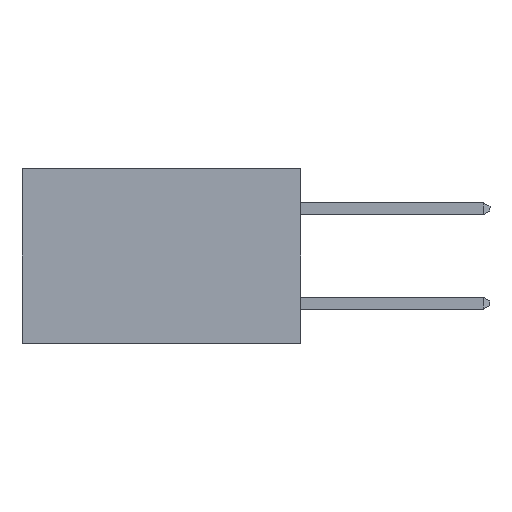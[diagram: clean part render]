
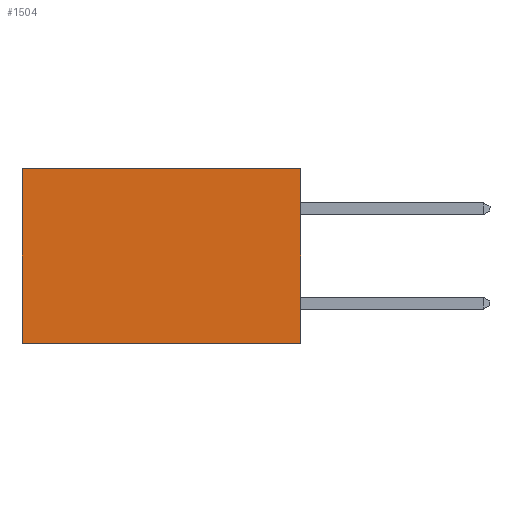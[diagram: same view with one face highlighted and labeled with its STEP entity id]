
A CAD part, left-side view. The second image highlights one B-rep face of the part: STEP entity #1504.
In plain terms, the highlighted planar face has unit normal (-1, 0, 0).
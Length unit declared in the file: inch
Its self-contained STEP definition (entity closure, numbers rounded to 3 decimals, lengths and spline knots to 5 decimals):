
#148 = VECTOR ( 'NONE', #6939, 39.37008 ) ;
#310 = VECTOR ( 'NONE', #2291, 39.37008 ) ;
#412 = ORIENTED_EDGE ( 'NONE', *, *, #3714, .T. ) ;
#515 = LINE ( 'NONE', #3896, #7092 ) ;
#741 = LINE ( 'NONE', #1169, #7304 ) ;
#976 = DIRECTION ( 'NONE',  ( 0., 1., 0. ) ) ;
#1053 = DIRECTION ( 'NONE',  ( 0., 0., -1. ) ) ;
#1169 = CARTESIAN_POINT ( 'NONE',  ( 0.277, 0., -0.37 ) ) ;
#1297 = DIRECTION ( 'NONE',  ( 0., 0., -1. ) ) ;
#1337 = DIRECTION ( 'NONE',  ( 1., 0., 0. ) ) ;
#1363 = PLANE ( 'NONE',  #7190 ) ;
#1504 = ADVANCED_FACE ( 'NONE', ( #4090 ), #1363, .F. ) ;
#1715 = CARTESIAN_POINT ( 'NONE',  ( 0.277, 0., -0.37 ) ) ;
#1769 = CARTESIAN_POINT ( 'NONE',  ( 0.277, 0., -0.37 ) ) ;
#1957 = EDGE_CURVE ( 'NONE', #2985, #2494, #741, .T. ) ;
#2291 = DIRECTION ( 'NONE',  ( 0., 1., 0. ) ) ;
#2494 = VERTEX_POINT ( 'NONE', #1769 ) ;
#2717 = VERTEX_POINT ( 'NONE', #8115 ) ;
#2786 = EDGE_CURVE ( 'NONE', #2717, #3017, #4804, .T. ) ;
#2985 = VERTEX_POINT ( 'NONE', #4842 ) ;
#3017 = VERTEX_POINT ( 'NONE', #4773 ) ;
#3580 = CARTESIAN_POINT ( 'NONE',  ( 0.277, 0., -0.37 ) ) ;
#3714 = EDGE_CURVE ( 'NONE', #2985, #2717, #515, .T. ) ;
#3896 = CARTESIAN_POINT ( 'NONE',  ( 0.277, 0., 0. ) ) ;
#4090 = FACE_OUTER_BOUND ( 'NONE', #5739, .T. ) ;
#4773 = CARTESIAN_POINT ( 'NONE',  ( 0.277, 0.59, -0.37 ) ) ;
#4804 = LINE ( 'NONE', #6836, #148 ) ;
#4832 = EDGE_CURVE ( 'NONE', #2494, #3017, #4989, .T. ) ;
#4842 = CARTESIAN_POINT ( 'NONE',  ( 0.277, 0., 0. ) ) ;
#4887 = ORIENTED_EDGE ( 'NONE', *, *, #4832, .F. ) ;
#4989 = LINE ( 'NONE', #3580, #310 ) ;
#5739 = EDGE_LOOP ( 'NONE', ( #7811, #4887, #6584, #412 ) ) ;
#6584 = ORIENTED_EDGE ( 'NONE', *, *, #1957, .F. ) ;
#6836 = CARTESIAN_POINT ( 'NONE',  ( 0.277, 0.59, -0.37 ) ) ;
#6939 = DIRECTION ( 'NONE',  ( 0., 0., -1. ) ) ;
#7092 = VECTOR ( 'NONE', #976, 39.37008 ) ;
#7190 = AXIS2_PLACEMENT_3D ( 'NONE', #1715, #1337, #1297 ) ;
#7304 = VECTOR ( 'NONE', #1053, 39.37008 ) ;
#7811 = ORIENTED_EDGE ( 'NONE', *, *, #2786, .T. ) ;
#8115 = CARTESIAN_POINT ( 'NONE',  ( 0.277, 0.59, 0. ) ) ;
